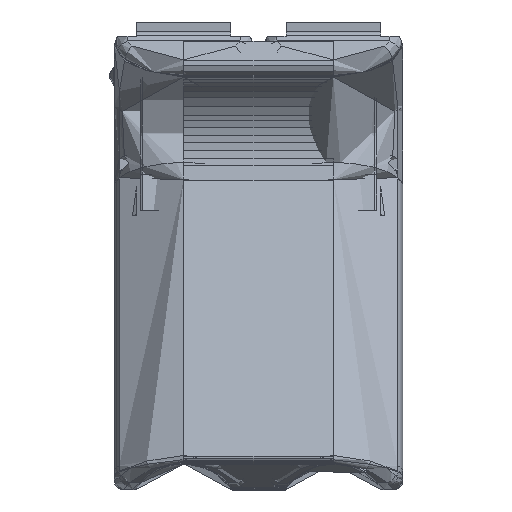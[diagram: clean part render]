
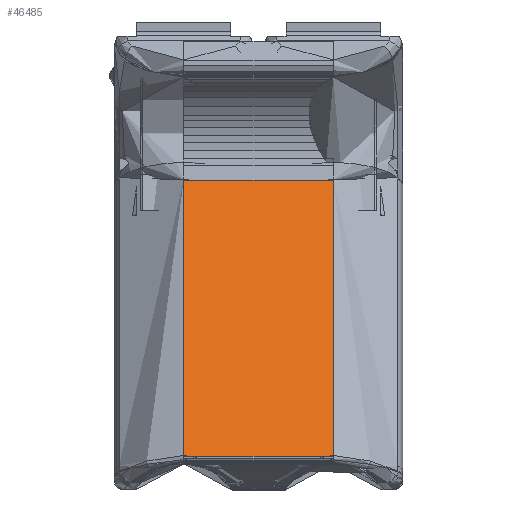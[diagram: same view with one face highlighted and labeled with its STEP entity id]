
A CAD part, left-side view. The second image highlights one B-rep face of the part: STEP entity #46485.
In plain terms, the highlighted planar face has unit normal (-0.931, 0, 0.366).
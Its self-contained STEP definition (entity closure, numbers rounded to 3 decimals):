
#6751=FACE_OUTER_BOUND('',#9320,.T.);
#9320=EDGE_LOOP('',(#41421,#41422,#41423,#41424));
#12615=LINE('',#143538,#16473);
#12638=LINE('',#143583,#16496);
#12701=LINE('',#143709,#16559);
#12702=LINE('',#143711,#16560);
#16473=VECTOR('',#58500,10.);
#16496=VECTOR('',#58531,10.);
#16559=VECTOR('',#58664,10.);
#16560=VECTOR('',#58667,10.);
#21312=VERTEX_POINT('',#143535);
#21313=VERTEX_POINT('',#143537);
#21330=VERTEX_POINT('',#143580);
#21331=VERTEX_POINT('',#143582);
#28045=EDGE_CURVE('',#21312,#21313,#12615,.T.);
#28068=EDGE_CURVE('',#21331,#21330,#12638,.T.);
#28131=EDGE_CURVE('',#21330,#21313,#12701,.T.);
#28132=EDGE_CURVE('',#21331,#21312,#12702,.T.);
#41421=ORIENTED_EDGE('',*,*,#28068,.T.);
#41422=ORIENTED_EDGE('',*,*,#28131,.T.);
#41423=ORIENTED_EDGE('',*,*,#28045,.F.);
#41424=ORIENTED_EDGE('',*,*,#28132,.F.);
#43981=PLANE('',#49634);
#46485=ADVANCED_FACE('',(#6751),#43981,.T.);
#49634=AXIS2_PLACEMENT_3D('',#143710,#58665,#58666);
#58500=DIRECTION('',(-0.366,0.,-0.931));
#58531=DIRECTION('',(-0.366,0.,-0.931));
#58664=DIRECTION('',(0.,-1.,0.));
#58665=DIRECTION('center_axis',(-0.931,0.,0.366));
#58666=DIRECTION('ref_axis',(-0.366,0.,-0.931));
#58667=DIRECTION('',(0.,-1.,0.));
#143535=CARTESIAN_POINT('',(11.668,-60.091,26.617));
#143537=CARTESIAN_POINT('',(-10.832,-60.091,-30.583));
#143538=CARTESIAN_POINT('',(11.668,-60.091,26.617));
#143580=CARTESIAN_POINT('',(-10.832,-29.091,-30.583));
#143582=CARTESIAN_POINT('',(11.668,-29.091,26.617));
#143583=CARTESIAN_POINT('',(11.668,-29.091,26.617));
#143709=CARTESIAN_POINT('',(-10.832,-29.091,-30.583));
#143710=CARTESIAN_POINT('Origin',(11.668,-29.091,26.617));
#143711=CARTESIAN_POINT('',(11.668,-29.091,26.617));
